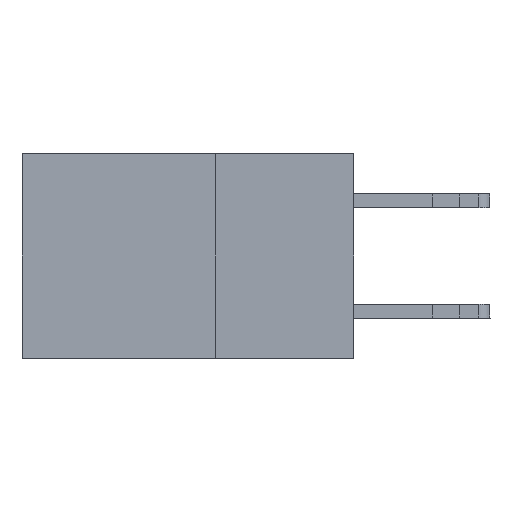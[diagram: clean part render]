
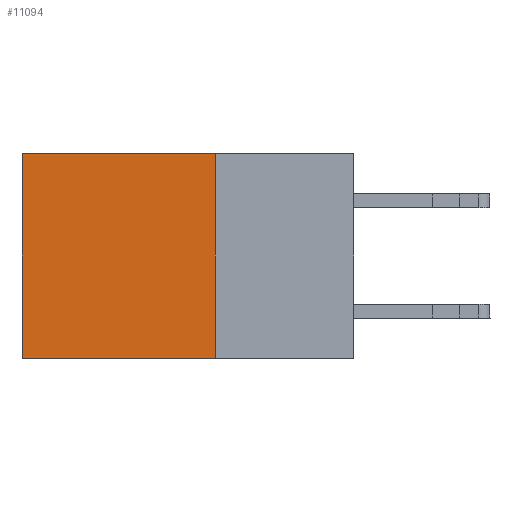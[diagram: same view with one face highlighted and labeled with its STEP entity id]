
A CAD part, left-side view. The second image highlights one B-rep face of the part: STEP entity #11094.
In plain terms, the highlighted planar face has unit normal (-1, 0, 0).
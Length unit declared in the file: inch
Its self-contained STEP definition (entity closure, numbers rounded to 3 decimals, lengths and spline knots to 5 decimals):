
#365 = AXIS2_PLACEMENT_3D ( 'NONE', #7466, #19805, #9224 ) ;
#1133 = CARTESIAN_POINT ( 'NONE',  ( 0.2875, 0.6, 0. ) ) ;
#1616 = FACE_OUTER_BOUND ( 'NONE', #1709, .T. ) ;
#1709 = EDGE_LOOP ( 'NONE', ( #5663, #18870, #14984, #8388 ) ) ;
#2039 = CARTESIAN_POINT ( 'NONE',  ( 0.2875, 0.6, 0. ) ) ;
#4660 = CARTESIAN_POINT ( 'NONE',  ( 0.2875, 0.25, -0.37 ) ) ;
#5460 = CARTESIAN_POINT ( 'NONE',  ( 0.2875, 0.6, -0.37 ) ) ;
#5663 = ORIENTED_EDGE ( 'NONE', *, *, #19511, .T. ) ;
#6094 = VECTOR ( 'NONE', #11830, 39.37008 ) ;
#7466 = CARTESIAN_POINT ( 'NONE',  ( 0.2875, 0.25, 0. ) ) ;
#7855 = CARTESIAN_POINT ( 'NONE',  ( 0.2875, 0.25, 0. ) ) ;
#7918 = LINE ( 'NONE', #7855, #20916 ) ;
#8388 = ORIENTED_EDGE ( 'NONE', *, *, #11695, .T. ) ;
#8592 = VERTEX_POINT ( 'NONE', #2039 ) ;
#9224 = DIRECTION ( 'NONE',  ( 0., 0., -1. ) ) ;
#10278 = LINE ( 'NONE', #1133, #6094 ) ;
#10954 = PLANE ( 'NONE',  #365 ) ;
#11094 = ADVANCED_FACE ( 'NONE', ( #1616 ), #10954, .F. ) ;
#11375 = CARTESIAN_POINT ( 'NONE',  ( 0.2875, 0.25, 0. ) ) ;
#11695 = EDGE_CURVE ( 'NONE', #13559, #8592, #17151, .T. ) ;
#11830 = DIRECTION ( 'NONE',  ( 0., 0., -1. ) ) ;
#13387 = DIRECTION ( 'NONE',  ( 0., 1., 0. ) ) ;
#13559 = VERTEX_POINT ( 'NONE', #11375 ) ;
#14158 = CARTESIAN_POINT ( 'NONE',  ( 0.2875, 0.25, -0.37 ) ) ;
#14286 = EDGE_CURVE ( 'NONE', #22584, #14852, #18549, .T. ) ;
#14852 = VERTEX_POINT ( 'NONE', #5460 ) ;
#14984 = ORIENTED_EDGE ( 'NONE', *, *, #22883, .F. ) ;
#17151 = LINE ( 'NONE', #22175, #21854 ) ;
#17992 = VECTOR ( 'NONE', #18820, 39.37008 ) ;
#18549 = LINE ( 'NONE', #4660, #17992 ) ;
#18820 = DIRECTION ( 'NONE',  ( 0., 1., 0. ) ) ;
#18870 = ORIENTED_EDGE ( 'NONE', *, *, #14286, .F. ) ;
#19511 = EDGE_CURVE ( 'NONE', #8592, #14852, #10278, .T. ) ;
#19805 = DIRECTION ( 'NONE',  ( 1., 0., 0. ) ) ;
#20916 = VECTOR ( 'NONE', #21982, 39.37008 ) ;
#21854 = VECTOR ( 'NONE', #13387, 39.37008 ) ;
#21982 = DIRECTION ( 'NONE',  ( 0., 0., -1. ) ) ;
#22175 = CARTESIAN_POINT ( 'NONE',  ( 0.2875, 0.25, 0. ) ) ;
#22584 = VERTEX_POINT ( 'NONE', #14158 ) ;
#22883 = EDGE_CURVE ( 'NONE', #13559, #22584, #7918, .T. ) ;
